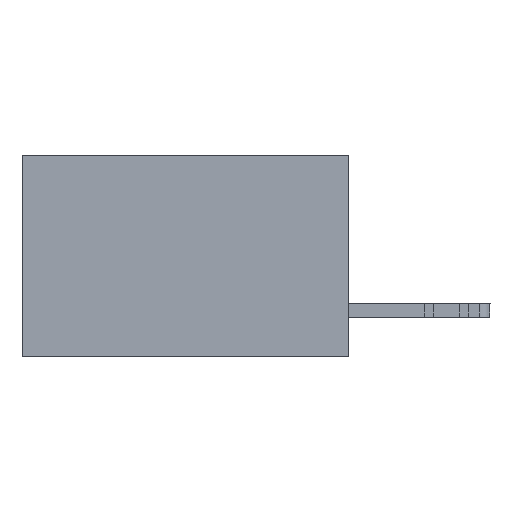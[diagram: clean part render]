
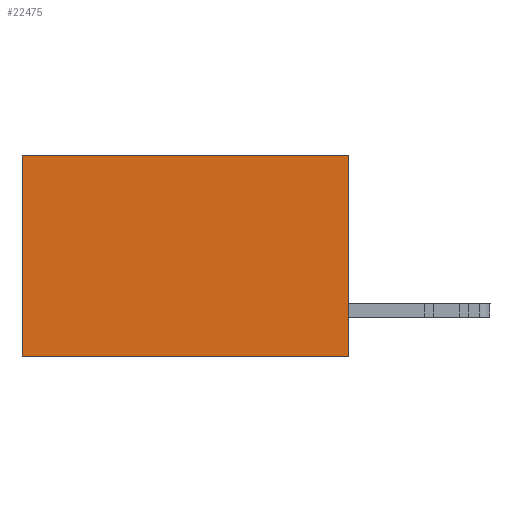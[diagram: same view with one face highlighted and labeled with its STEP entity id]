
A CAD part, left-side view. The second image highlights one B-rep face of the part: STEP entity #22475.
In plain terms, the highlighted planar face has unit normal (-1, 0, 0).
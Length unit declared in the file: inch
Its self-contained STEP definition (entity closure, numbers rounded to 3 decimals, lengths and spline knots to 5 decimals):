
#1010 = EDGE_LOOP ( 'NONE', ( #9694, #4544, #21792, #12698 ) ) ;
#1957 = VERTEX_POINT ( 'NONE', #14123 ) ;
#2085 = EDGE_CURVE ( 'NONE', #22647, #14124, #12992, .T. ) ;
#2191 = DIRECTION ( 'NONE',  ( 0., 1., 0. ) ) ;
#2985 = VECTOR ( 'NONE', #11887, 39.37008 ) ;
#4544 = ORIENTED_EDGE ( 'NONE', *, *, #9678, .F. ) ;
#5201 = EDGE_CURVE ( 'NONE', #10630, #1957, #9432, .T. ) ;
#5862 = CARTESIAN_POINT ( 'NONE',  ( 0.2615, 0.6, 0. ) ) ;
#5884 = LINE ( 'NONE', #9966, #11930 ) ;
#7126 = DIRECTION ( 'NONE',  ( 0., 0., -1. ) ) ;
#7710 = AXIS2_PLACEMENT_3D ( 'NONE', #22018, #24005, #7126 ) ;
#8217 = DIRECTION ( 'NONE',  ( 0., 1., 0. ) ) ;
#9342 = CARTESIAN_POINT ( 'NONE',  ( 0.2615, 0., 0. ) ) ;
#9432 = LINE ( 'NONE', #18903, #2985 ) ;
#9678 = EDGE_CURVE ( 'NONE', #1957, #14124, #18388, .T. ) ;
#9694 = ORIENTED_EDGE ( 'NONE', *, *, #2085, .T. ) ;
#9966 = CARTESIAN_POINT ( 'NONE',  ( 0.2615, 0., 0. ) ) ;
#10630 = VERTEX_POINT ( 'NONE', #9342 ) ;
#11887 = DIRECTION ( 'NONE',  ( 0., 0., -1. ) ) ;
#11930 = VECTOR ( 'NONE', #2191, 39.37008 ) ;
#12698 = ORIENTED_EDGE ( 'NONE', *, *, #23868, .T. ) ;
#12927 = CARTESIAN_POINT ( 'NONE',  ( 0.2615, 0.6, -0.37 ) ) ;
#12992 = LINE ( 'NONE', #20498, #14709 ) ;
#14123 = CARTESIAN_POINT ( 'NONE',  ( 0.2615, 0., -0.37 ) ) ;
#14124 = VERTEX_POINT ( 'NONE', #12927 ) ;
#14709 = VECTOR ( 'NONE', #20382, 39.37008 ) ;
#16508 = PLANE ( 'NONE',  #7710 ) ;
#18388 = LINE ( 'NONE', #20115, #22337 ) ;
#18903 = CARTESIAN_POINT ( 'NONE',  ( 0.2615, 0., -0.37 ) ) ;
#20115 = CARTESIAN_POINT ( 'NONE',  ( 0.2615, 0., -0.37 ) ) ;
#20382 = DIRECTION ( 'NONE',  ( 0., 0., -1. ) ) ;
#20439 = FACE_OUTER_BOUND ( 'NONE', #1010, .T. ) ;
#20498 = CARTESIAN_POINT ( 'NONE',  ( 0.2615, 0.6, -0.37 ) ) ;
#21792 = ORIENTED_EDGE ( 'NONE', *, *, #5201, .F. ) ;
#22018 = CARTESIAN_POINT ( 'NONE',  ( 0.2615, 0., -0.37 ) ) ;
#22337 = VECTOR ( 'NONE', #8217, 39.37008 ) ;
#22475 = ADVANCED_FACE ( 'NONE', ( #20439 ), #16508, .F. ) ;
#22647 = VERTEX_POINT ( 'NONE', #5862 ) ;
#23868 = EDGE_CURVE ( 'NONE', #10630, #22647, #5884, .T. ) ;
#24005 = DIRECTION ( 'NONE',  ( 1., 0., 0. ) ) ;
